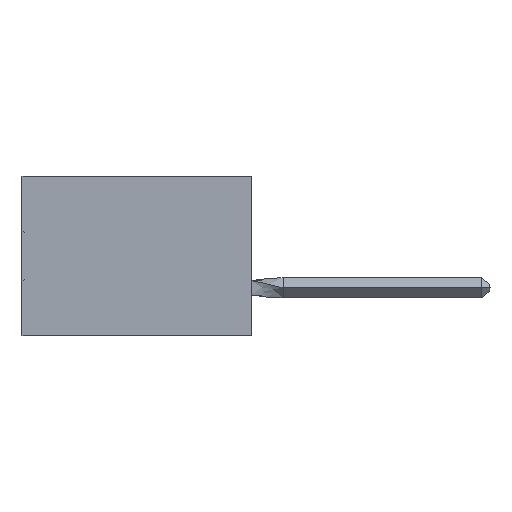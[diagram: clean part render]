
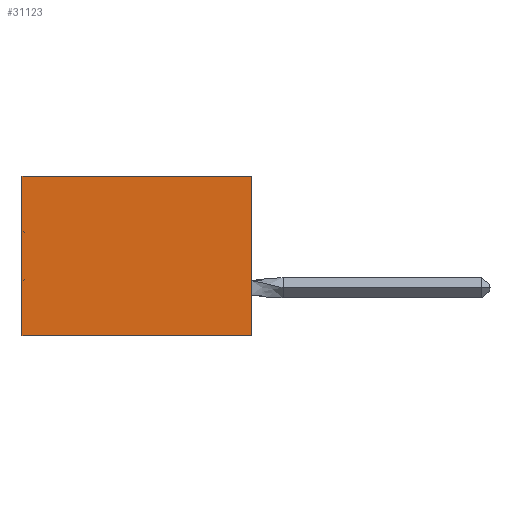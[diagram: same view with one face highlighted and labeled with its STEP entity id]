
A CAD part, left-side view. The second image highlights one B-rep face of the part: STEP entity #31123.
In plain terms, the highlighted planar face has unit normal (-1, 0, 0).
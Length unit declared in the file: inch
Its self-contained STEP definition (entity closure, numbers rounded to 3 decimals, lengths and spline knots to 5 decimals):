
#2420 = VERTEX_POINT ( 'NONE', #43736 ) ;
#4767 = AXIS2_PLACEMENT_3D ( 'NONE', #16160, #57248, #34541 ) ;
#6986 = LINE ( 'NONE', #58898, #39089 ) ;
#8300 = LINE ( 'NONE', #19481, #48239 ) ;
#12092 = EDGE_CURVE ( 'NONE', #14238, #39216, #41957, .T. ) ;
#12863 = EDGE_CURVE ( 'NONE', #2420, #13736, #8300, .T. ) ;
#13222 = DIRECTION ( 'NONE',  ( 0., 0., -1. ) ) ;
#13736 = VERTEX_POINT ( 'NONE', #39809 ) ;
#14238 = VERTEX_POINT ( 'NONE', #19875 ) ;
#14258 = CARTESIAN_POINT ( 'NONE',  ( 0.305, 0., -0.5 ) ) ;
#14937 = DIRECTION ( 'NONE',  ( 0., 0., -1. ) ) ;
#16160 = CARTESIAN_POINT ( 'NONE',  ( 0.305, 0., -0.5 ) ) ;
#16995 = CARTESIAN_POINT ( 'NONE',  ( 0.305, 0., -0.5 ) ) ;
#19481 = CARTESIAN_POINT ( 'NONE',  ( 0.305, 0.72, -0.5 ) ) ;
#19875 = CARTESIAN_POINT ( 'NONE',  ( 0.305, 0., 0. ) ) ;
#19945 = LINE ( 'NONE', #34819, #22123 ) ;
#22123 = VECTOR ( 'NONE', #52891, 39.37008 ) ;
#27811 = VECTOR ( 'NONE', #13222, 39.37008 ) ;
#31123 = ADVANCED_FACE ( 'NONE', ( #38966 ), #43435, .F. ) ;
#33188 = EDGE_LOOP ( 'NONE', ( #52324, #46428, #48433, #47810 ) ) ;
#34541 = DIRECTION ( 'NONE',  ( 0., 0., -1. ) ) ;
#34819 = CARTESIAN_POINT ( 'NONE',  ( 0.305, 0., 0. ) ) ;
#36197 = DIRECTION ( 'NONE',  ( 0., 1., 0. ) ) ;
#38966 = FACE_OUTER_BOUND ( 'NONE', #33188, .T. ) ;
#39089 = VECTOR ( 'NONE', #36197, 39.37008 ) ;
#39216 = VERTEX_POINT ( 'NONE', #14258 ) ;
#39809 = CARTESIAN_POINT ( 'NONE',  ( 0.305, 0.72, -0.5 ) ) ;
#41957 = LINE ( 'NONE', #16995, #27811 ) ;
#43435 = PLANE ( 'NONE',  #4767 ) ;
#43736 = CARTESIAN_POINT ( 'NONE',  ( 0.305, 0.72, 0. ) ) ;
#46428 = ORIENTED_EDGE ( 'NONE', *, *, #50718, .F. ) ;
#47810 = ORIENTED_EDGE ( 'NONE', *, *, #57951, .T. ) ;
#48239 = VECTOR ( 'NONE', #14937, 39.37008 ) ;
#48433 = ORIENTED_EDGE ( 'NONE', *, *, #12092, .F. ) ;
#50718 = EDGE_CURVE ( 'NONE', #39216, #13736, #6986, .T. ) ;
#52324 = ORIENTED_EDGE ( 'NONE', *, *, #12863, .T. ) ;
#52891 = DIRECTION ( 'NONE',  ( 0., 1., 0. ) ) ;
#57248 = DIRECTION ( 'NONE',  ( 1., 0., 0. ) ) ;
#57951 = EDGE_CURVE ( 'NONE', #14238, #2420, #19945, .T. ) ;
#58898 = CARTESIAN_POINT ( 'NONE',  ( 0.305, 0., -0.5 ) ) ;
